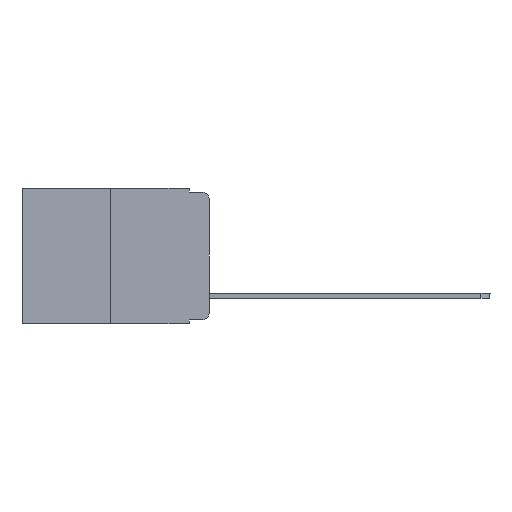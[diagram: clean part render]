
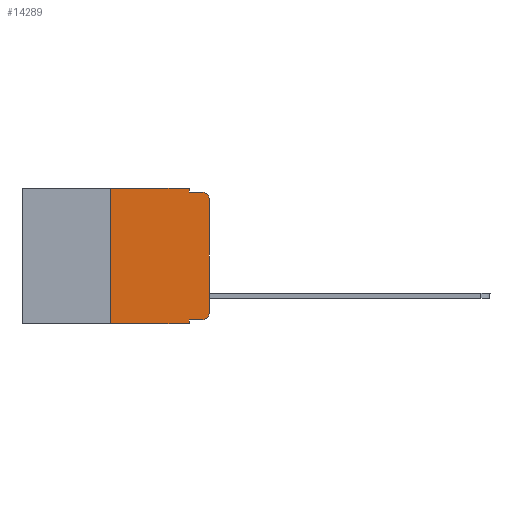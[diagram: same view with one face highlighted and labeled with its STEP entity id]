
A CAD part, left-side view. The second image highlights one B-rep face of the part: STEP entity #14289.
In plain terms, the highlighted planar face has unit normal (-1, 0, 0).
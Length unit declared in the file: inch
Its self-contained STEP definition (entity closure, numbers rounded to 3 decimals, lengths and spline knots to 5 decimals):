
#538 = VERTEX_POINT ( 'NONE', #13728 ) ;
#785 = VECTOR ( 'NONE', #10448, 39.37008 ) ;
#855 = CARTESIAN_POINT ( 'NONE',  ( 0., 0.25, 0. ) ) ;
#965 = ORIENTED_EDGE ( 'NONE', *, *, #4655, .T. ) ;
#1438 = VERTEX_POINT ( 'NONE', #13555 ) ;
#1445 = CARTESIAN_POINT ( 'NONE',  ( 0., 0.051, 0. ) ) ;
#1682 = ORIENTED_EDGE ( 'NONE', *, *, #23460, .T. ) ;
#2626 = CARTESIAN_POINT ( 'NONE',  ( 0., 0.02, -0.313 ) ) ;
#2634 = CARTESIAN_POINT ( 'NONE',  ( 0., 0., 0. ) ) ;
#3156 = CARTESIAN_POINT ( 'NONE',  ( 0., 0.02, -0.03 ) ) ;
#3598 = CARTESIAN_POINT ( 'NONE',  ( 0., 0.25, -0.343 ) ) ;
#3679 = CIRCLE ( 'NONE', #17629, 0.02 ) ;
#3903 = CARTESIAN_POINT ( 'NONE',  ( 0., 0., -0.313 ) ) ;
#4105 = EDGE_CURVE ( 'NONE', #11208, #12741, #23865, .T. ) ;
#4220 = EDGE_CURVE ( 'NONE', #538, #19227, #22980, .T. ) ;
#4408 = DIRECTION ( 'NONE',  ( -1., 0., 0. ) ) ;
#4481 = DIRECTION ( 'NONE',  ( 0., -1., 0. ) ) ;
#4590 = DIRECTION ( 'NONE',  ( 0., 0., -1. ) ) ;
#4649 = EDGE_CURVE ( 'NONE', #7610, #7266, #10916, .T. ) ;
#4655 = EDGE_CURVE ( 'NONE', #11241, #11208, #21134, .T. ) ;
#5270 = ORIENTED_EDGE ( 'NONE', *, *, #4649, .F. ) ;
#5599 = AXIS2_PLACEMENT_3D ( 'NONE', #16290, #17960, #4590 ) ;
#5662 = ORIENTED_EDGE ( 'NONE', *, *, #18008, .F. ) ;
#5919 = FACE_OUTER_BOUND ( 'NONE', #8020, .T. ) ;
#6166 = DIRECTION ( 'NONE',  ( 0., 0., -1. ) ) ;
#6783 = DIRECTION ( 'NONE',  ( -1., 0., 0. ) ) ;
#7266 = VERTEX_POINT ( 'NONE', #21133 ) ;
#7610 = VERTEX_POINT ( 'NONE', #3598 ) ;
#8020 = EDGE_LOOP ( 'NONE', ( #965, #19438, #9403, #5662, #22428, #5270, #1682, #8309, #16549, #20606 ) ) ;
#8309 = ORIENTED_EDGE ( 'NONE', *, *, #14387, .F. ) ;
#8628 = DIRECTION ( 'NONE',  ( 0., -1., 0. ) ) ;
#8887 = CARTESIAN_POINT ( 'NONE',  ( 0., 0.051, 0. ) ) ;
#9218 = DIRECTION ( 'NONE',  ( 0., -1., 0. ) ) ;
#9403 = ORIENTED_EDGE ( 'NONE', *, *, #14859, .F. ) ;
#9436 = VECTOR ( 'NONE', #16881, 39.37008 ) ;
#10448 = DIRECTION ( 'NONE',  ( 0., -1., 0. ) ) ;
#10916 = LINE ( 'NONE', #855, #20536 ) ;
#11208 = VERTEX_POINT ( 'NONE', #18988 ) ;
#11241 = VERTEX_POINT ( 'NONE', #3903 ) ;
#11471 = VERTEX_POINT ( 'NONE', #22081 ) ;
#12141 = CARTESIAN_POINT ( 'NONE',  ( 0., 0.473, -0.343 ) ) ;
#12159 = PLANE ( 'NONE',  #5599 ) ;
#12298 = CARTESIAN_POINT ( 'NONE',  ( 0., 0.051, -0.01 ) ) ;
#12382 = CARTESIAN_POINT ( 'NONE',  ( 0., 0.02, -0.333 ) ) ;
#12586 = LINE ( 'NONE', #20242, #19781 ) ;
#12741 = VERTEX_POINT ( 'NONE', #20175 ) ;
#13555 = CARTESIAN_POINT ( 'NONE',  ( 0., 0.051, -0.343 ) ) ;
#13728 = CARTESIAN_POINT ( 'NONE',  ( 0., 0.051, -0.333 ) ) ;
#14289 = ADVANCED_FACE ( 'NONE', ( #5919 ), #12159, .F. ) ;
#14344 = CARTESIAN_POINT ( 'NONE',  ( 0., 0.473, 0. ) ) ;
#14387 = EDGE_CURVE ( 'NONE', #538, #1438, #12586, .T. ) ;
#14554 = LINE ( 'NONE', #8887, #9436 ) ;
#14686 = VECTOR ( 'NONE', #8628, 39.37008 ) ;
#14859 = EDGE_CURVE ( 'NONE', #11471, #12741, #15570, .T. ) ;
#15008 = VECTOR ( 'NONE', #4481, 39.37008 ) ;
#15570 = LINE ( 'NONE', #12298, #785 ) ;
#16290 = CARTESIAN_POINT ( 'NONE',  ( 0., 0.473, 0. ) ) ;
#16549 = ORIENTED_EDGE ( 'NONE', *, *, #4220, .T. ) ;
#16550 = DIRECTION ( 'NONE',  ( 0., 0., -1. ) ) ;
#16881 = DIRECTION ( 'NONE',  ( 0., 0., -1. ) ) ;
#17629 = AXIS2_PLACEMENT_3D ( 'NONE', #2626, #4408, #6166 ) ;
#17960 = DIRECTION ( 'NONE',  ( 1., 0., 0. ) ) ;
#18008 = EDGE_CURVE ( 'NONE', #19107, #11471, #14554, .T. ) ;
#18457 = DIRECTION ( 'NONE',  ( 0., 0., -1. ) ) ;
#18494 = EDGE_CURVE ( 'NONE', #19227, #11241, #3679, .T. ) ;
#18988 = CARTESIAN_POINT ( 'NONE',  ( 0., 0., -0.03 ) ) ;
#19107 = VERTEX_POINT ( 'NONE', #1445 ) ;
#19227 = VERTEX_POINT ( 'NONE', #12382 ) ;
#19438 = ORIENTED_EDGE ( 'NONE', *, *, #4105, .T. ) ;
#19472 = AXIS2_PLACEMENT_3D ( 'NONE', #3156, #6783, #16550 ) ;
#19781 = VECTOR ( 'NONE', #18457, 39.37008 ) ;
#20119 = LINE ( 'NONE', #12141, #15008 ) ;
#20175 = CARTESIAN_POINT ( 'NONE',  ( 0., 0.02, -0.01 ) ) ;
#20236 = DIRECTION ( 'NONE',  ( 0., 0., 1. ) ) ;
#20242 = CARTESIAN_POINT ( 'NONE',  ( 0., 0.051, 0. ) ) ;
#20536 = VECTOR ( 'NONE', #20236, 39.37008 ) ;
#20606 = ORIENTED_EDGE ( 'NONE', *, *, #18494, .T. ) ;
#21133 = CARTESIAN_POINT ( 'NONE',  ( 0., 0.25, 0. ) ) ;
#21134 = LINE ( 'NONE', #2634, #22954 ) ;
#21778 = EDGE_CURVE ( 'NONE', #7266, #19107, #22212, .T. ) ;
#22081 = CARTESIAN_POINT ( 'NONE',  ( 0., 0.051, -0.01 ) ) ;
#22212 = LINE ( 'NONE', #14344, #14686 ) ;
#22428 = ORIENTED_EDGE ( 'NONE', *, *, #21778, .F. ) ;
#22764 = CARTESIAN_POINT ( 'NONE',  ( 0., 0.051, -0.333 ) ) ;
#22954 = VECTOR ( 'NONE', #24011, 39.37008 ) ;
#22980 = LINE ( 'NONE', #22764, #23270 ) ;
#23270 = VECTOR ( 'NONE', #9218, 39.37008 ) ;
#23460 = EDGE_CURVE ( 'NONE', #7610, #1438, #20119, .T. ) ;
#23865 = CIRCLE ( 'NONE', #19472, 0.02 ) ;
#24011 = DIRECTION ( 'NONE',  ( 0., 0., 1. ) ) ;
